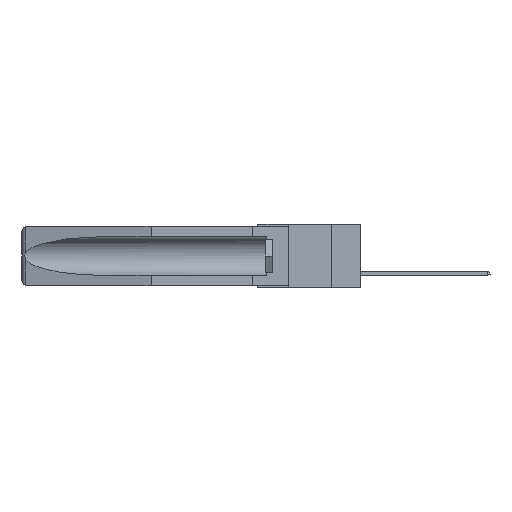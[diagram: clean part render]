
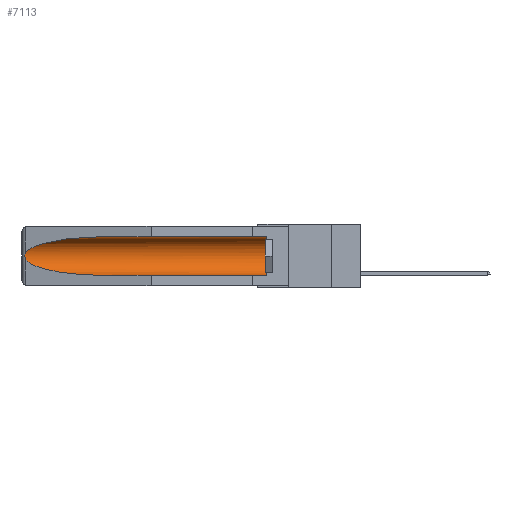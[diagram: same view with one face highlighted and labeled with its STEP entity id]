
A CAD part, left-side view. The second image highlights one B-rep face of the part: STEP entity #7113.
In plain terms, the highlighted cylindrical face has radius 2.857 mm (diameter 5.715 mm), a partial arc.
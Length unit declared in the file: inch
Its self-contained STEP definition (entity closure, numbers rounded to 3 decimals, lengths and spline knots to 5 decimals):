
#161 = LINE ( 'NONE', #8836, #11133 ) ;
#682 = EDGE_LOOP ( 'NONE', ( #21049, #3743, #5946, #10044, #20029, #3141 ) ) ;
#1367 = VERTEX_POINT ( 'NONE', #13735 ) ;
#1428 = CARTESIAN_POINT ( 'NONE',  ( 0.26654, 1.53092, -0.15636 ) ) ;
#1615 = CARTESIAN_POINT ( 'NONE',  ( 0.26597, 1.5296, -0.19026 ) ) ;
#1739 = VECTOR ( 'NONE', #4377, 39.37008 ) ;
#1813 = CARTESIAN_POINT ( 'NONE',  ( 0.2675, 1.53308, -0.16763 ) ) ;
#2070 = CARTESIAN_POINT ( 'NONE',  ( 0.155, 1.07973, -0.059 ) ) ;
#2348 = EDGE_CURVE ( 'NONE', #9714, #28112, #23779, .T. ) ;
#2450 = CARTESIAN_POINT ( 'NONE',  ( 0.155, -0.30754, -0.284 ) ) ;
#3141 = ORIENTED_EDGE ( 'NONE', *, *, #5290, .T. ) ;
#3341 = CARTESIAN_POINT ( 'NONE',  ( 0.25451, 1.48313, -0.24835 ) ) ;
#3608 = DIRECTION ( 'NONE',  ( 0., -1., 0. ) ) ;
#3609 = CARTESIAN_POINT ( 'NONE',  ( 0.2675, 1.53308, -0.17534 ) ) ;
#3621 = CARTESIAN_POINT ( 'NONE',  ( 0.155, 1.07973, -0.284 ) ) ;
#3743 = ORIENTED_EDGE ( 'NONE', *, *, #2348, .T. ) ;
#4121 = VERTEX_POINT ( 'NONE', #25224 ) ;
#4330 = AXIS2_PLACEMENT_3D ( 'NONE', #25924, #8416, #15038 ) ;
#4377 = DIRECTION ( 'NONE',  ( 0., 1., 0. ) ) ;
#5290 = EDGE_CURVE ( 'NONE', #1367, #25399, #161, .T. ) ;
#5946 = ORIENTED_EDGE ( 'NONE', *, *, #17052, .T. ) ;
#5967 = CARTESIAN_POINT ( 'NONE',  ( 0.26537, 1.52718, -0.19328 ) ) ;
#6605 = CARTESIAN_POINT ( 'NONE',  ( 0.26537, 1.52718, -0.14972 ) ) ;
#7113 = ADVANCED_FACE ( 'NONE', ( #16815 ), #21261, .F. ) ;
#8416 = DIRECTION ( 'NONE',  ( 0., 1., 0. ) ) ;
#8836 = CARTESIAN_POINT ( 'NONE',  ( 0.155, -0.30754, -0.059 ) ) ;
#9714 = VERTEX_POINT ( 'NONE', #11301 ) ;
#10044 = ORIENTED_EDGE ( 'NONE', *, *, #13881, .F. ) ;
#11133 = VECTOR ( 'NONE', #13294, 39.37008 ) ;
#11301 = CARTESIAN_POINT ( 'NONE',  ( 0.26537, 1.52718, -0.14972 ) ) ;
#11327 = VERTEX_POINT ( 'NONE', #20715 ) ;
#12358 = CARTESIAN_POINT ( 'NONE',  ( 0.26597, 1.52961, -0.15275 ) ) ;
#12375 = CARTESIAN_POINT ( 'NONE',  ( 0.21114, 1.30732, -0.284 ) ) ;
#13294 = DIRECTION ( 'NONE',  ( 0., 1., 0. ) ) ;
#13735 = CARTESIAN_POINT ( 'NONE',  ( 0.155, 0.126, -0.059 ) ) ;
#13881 = EDGE_CURVE ( 'NONE', #11327, #4121, #17477, .T. ) ;
#14333 = AXIS2_PLACEMENT_3D ( 'NONE', #25409, #3608, #18803 ) ;
#14480 = EDGE_CURVE ( 'NONE', #11327, #1367, #23576, .T. ) ;
#15038 = DIRECTION ( 'NONE',  ( 0., 0., 1. ) ) ;
#15381 =( BOUNDED_CURVE ( )  B_SPLINE_CURVE ( 3, ( #5967, #3341, #12375, #3621 ),
 .UNSPECIFIED., .F., .F. ) 
 B_SPLINE_CURVE_WITH_KNOTS ( ( 4, 4 ),
 ( 0.1948, 1.5708 ),
 .UNSPECIFIED. ) 
 CURVE ( )  GEOMETRIC_REPRESENTATION_ITEM ( )  RATIONAL_B_SPLINE_CURVE ( ( 1., 0.848, 0.848, 1. ) ) 
 REPRESENTATION_ITEM ( '' )  );
#16815 = FACE_OUTER_BOUND ( 'NONE', #682, .T. ) ;
#16907 = CARTESIAN_POINT ( 'NONE',  ( 0.2673, 1.5327, -0.16383 ) ) ;
#17052 = EDGE_CURVE ( 'NONE', #28112, #4121, #15381, .T. ) ;
#17060 = CARTESIAN_POINT ( 'NONE',  ( 0.25451, 1.48313, -0.09465 ) ) ;
#17355 = CARTESIAN_POINT ( 'NONE',  ( 0.21114, 1.30732, -0.059 ) ) ;
#17477 = LINE ( 'NONE', #2450, #1739 ) ;
#18348 =( BOUNDED_CURVE ( )  B_SPLINE_CURVE ( 3, ( #2070, #17355, #17060, #6605 ),
 .UNSPECIFIED., .F., .F. ) 
 B_SPLINE_CURVE_WITH_KNOTS ( ( 4, 4 ),
 ( 4.71239, 6.08839 ),
 .UNSPECIFIED. ) 
 CURVE ( )  GEOMETRIC_REPRESENTATION_ITEM ( )  RATIONAL_B_SPLINE_CURVE ( ( 1., 0.848, 0.848, 1. ) ) 
 REPRESENTATION_ITEM ( '' )  );
#18803 = DIRECTION ( 'NONE',  ( 0., 0., 1. ) ) ;
#18998 = CARTESIAN_POINT ( 'NONE',  ( 0.26655, 1.53094, -0.18657 ) ) ;
#20029 = ORIENTED_EDGE ( 'NONE', *, *, #14480, .T. ) ;
#20715 = CARTESIAN_POINT ( 'NONE',  ( 0.155, 0.126, -0.284 ) ) ;
#21049 = ORIENTED_EDGE ( 'NONE', *, *, #23527, .T. ) ;
#21200 = CARTESIAN_POINT ( 'NONE',  ( 0.2673, 1.53269, -0.17917 ) ) ;
#21261 = CYLINDRICAL_SURFACE ( 'NONE', #4330, 0.1125 ) ;
#22797 = CARTESIAN_POINT ( 'NONE',  ( 0.155, 1.07973, -0.059 ) ) ;
#23527 = EDGE_CURVE ( 'NONE', #25399, #9714, #18348, .T. ) ;
#23576 = CIRCLE ( 'NONE', #14333, 0.1125 ) ;
#23779 = B_SPLINE_CURVE_WITH_KNOTS ( 'NONE', 3,
 ( #27792, #12358, #1428, #16907, #1813, #3609, #21200, #18998, #1615, #27883 ),
 .UNSPECIFIED., .F., .F.,
 ( 4, 2, 2, 2, 4 ),
 ( 0., 0.00029, 0.00058, 0.00087, 0.00117 ),
 .UNSPECIFIED. ) ;
#25128 = CARTESIAN_POINT ( 'NONE',  ( 0.26537, 1.52718, -0.19328 ) ) ;
#25224 = CARTESIAN_POINT ( 'NONE',  ( 0.155, 1.07973, -0.284 ) ) ;
#25399 = VERTEX_POINT ( 'NONE', #22797 ) ;
#25409 = CARTESIAN_POINT ( 'NONE',  ( 0.155, 0.126, -0.1715 ) ) ;
#25924 = CARTESIAN_POINT ( 'NONE',  ( 0.155, -0.30754, -0.1715 ) ) ;
#27792 = CARTESIAN_POINT ( 'NONE',  ( 0.26537, 1.52718, -0.14972 ) ) ;
#27883 = CARTESIAN_POINT ( 'NONE',  ( 0.26537, 1.52718, -0.19328 ) ) ;
#28112 = VERTEX_POINT ( 'NONE', #25128 ) ;
